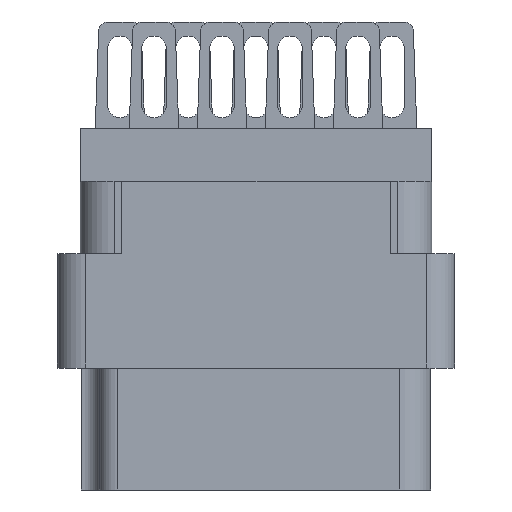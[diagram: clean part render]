
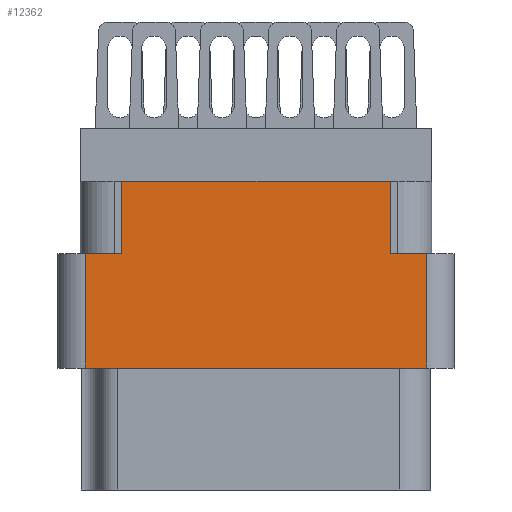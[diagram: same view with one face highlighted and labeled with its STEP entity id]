
A CAD part, left-side view. The second image highlights one B-rep face of the part: STEP entity #12362.
In plain terms, the highlighted planar face has unit normal (-1, 0, 0).
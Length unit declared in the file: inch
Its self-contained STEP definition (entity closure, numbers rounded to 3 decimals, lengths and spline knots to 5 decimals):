
#1433 = CARTESIAN_POINT ( 'NONE',  ( -1.296, 0., -0.277 ) ) ;
#1527 = VECTOR ( 'NONE', #34134, 39.37008 ) ;
#1602 = ORIENTED_EDGE ( 'NONE', *, *, #22828, .F. ) ;
#4025 = VECTOR ( 'NONE', #23517, 39.37008 ) ;
#4222 = DIRECTION ( 'NONE',  ( 0., -1., 0. ) ) ;
#6904 = VERTEX_POINT ( 'NONE', #41774 ) ;
#7557 = ORIENTED_EDGE ( 'NONE', *, *, #26108, .F. ) ;
#8446 = DIRECTION ( 'NONE',  ( -1., 0., 0. ) ) ;
#8701 = DIRECTION ( 'NONE',  ( 0., -1., 0. ) ) ;
#10532 = CARTESIAN_POINT ( 'NONE',  ( -1.296, 0.296, -0.277 ) ) ;
#11224 = LINE ( 'NONE', #1433, #1527 ) ;
#11901 = CARTESIAN_POINT ( 'NONE',  ( -1.296, -0.296, -0.117 ) ) ;
#12362 = ADVANCED_FACE ( 'NONE', ( #31519 ), #41620, .T. ) ;
#13215 = VECTOR ( 'NONE', #15807, 39.37008 ) ;
#15366 = EDGE_CURVE ( 'NONE', #37491, #18686, #37211, .T. ) ;
#15807 = DIRECTION ( 'NONE',  ( 0., 0., 1. ) ) ;
#16629 = ORIENTED_EDGE ( 'NONE', *, *, #15366, .T. ) ;
#18030 = ORIENTED_EDGE ( 'NONE', *, *, #46895, .F. ) ;
#18686 = VERTEX_POINT ( 'NONE', #47164 ) ;
#18992 = CARTESIAN_POINT ( 'NONE',  ( -1.296, 0.438, -0.117 ) ) ;
#20115 = VERTEX_POINT ( 'NONE', #20280 ) ;
#20280 = CARTESIAN_POINT ( 'NONE',  ( -1.296, -0.376, -0.529 ) ) ;
#20473 = LINE ( 'NONE', #41917, #4025 ) ;
#21093 = LINE ( 'NONE', #18992, #23906 ) ;
#21752 = CARTESIAN_POINT ( 'NONE',  ( -1.296, 0.296, -0.117 ) ) ;
#22828 = EDGE_CURVE ( 'NONE', #41515, #23823, #27057, .T. ) ;
#23211 = CARTESIAN_POINT ( 'NONE',  ( -1.296, -0.376, -0.277 ) ) ;
#23517 = DIRECTION ( 'NONE',  ( 0., 0., 1. ) ) ;
#23823 = VERTEX_POINT ( 'NONE', #21752 ) ;
#23906 = VECTOR ( 'NONE', #4222, 39.37008 ) ;
#25377 = ORIENTED_EDGE ( 'NONE', *, *, #26631, .T. ) ;
#26108 = EDGE_CURVE ( 'NONE', #37491, #41515, #35412, .T. ) ;
#26454 = VERTEX_POINT ( 'NONE', #23211 ) ;
#26631 = EDGE_CURVE ( 'NONE', #6904, #33984, #20473, .T. ) ;
#27057 = LINE ( 'NONE', #27490, #40815 ) ;
#27490 = CARTESIAN_POINT ( 'NONE',  ( -1.296, 0.296, -0.277 ) ) ;
#27792 = DIRECTION ( 'NONE',  ( 0., 0., -1. ) ) ;
#29045 = ORIENTED_EDGE ( 'NONE', *, *, #40742, .T. ) ;
#29537 = EDGE_CURVE ( 'NONE', #23823, #33984, #21093, .T. ) ;
#29660 = CARTESIAN_POINT ( 'NONE',  ( -1.296, -0.376, -0.798 ) ) ;
#30866 = VECTOR ( 'NONE', #27792, 39.37008 ) ;
#31105 = DIRECTION ( 'NONE',  ( 0., 1., 0. ) ) ;
#31111 = CARTESIAN_POINT ( 'NONE',  ( -1.296, 0., -0.277 ) ) ;
#31151 = DIRECTION ( 'NONE',  ( 0., 0., 1. ) ) ;
#31294 = AXIS2_PLACEMENT_3D ( 'NONE', #41465, #8446, #33954 ) ;
#31519 = FACE_OUTER_BOUND ( 'NONE', #43573, .T. ) ;
#32199 = LINE ( 'NONE', #38674, #34525 ) ;
#32902 = EDGE_CURVE ( 'NONE', #20115, #18686, #32199, .T. ) ;
#33954 = DIRECTION ( 'NONE',  ( 0., 0., 1. ) ) ;
#33984 = VERTEX_POINT ( 'NONE', #11901 ) ;
#34134 = DIRECTION ( 'NONE',  ( 0., -1., 0. ) ) ;
#34525 = VECTOR ( 'NONE', #31105, 39.37008 ) ;
#35412 = LINE ( 'NONE', #31111, #37161 ) ;
#37161 = VECTOR ( 'NONE', #8701, 39.37008 ) ;
#37211 = LINE ( 'NONE', #39186, #30866 ) ;
#37491 = VERTEX_POINT ( 'NONE', #44864 ) ;
#38674 = CARTESIAN_POINT ( 'NONE',  ( -1.296, 0., -0.529 ) ) ;
#39186 = CARTESIAN_POINT ( 'NONE',  ( -1.296, 0.376, -0.798 ) ) ;
#40742 = EDGE_CURVE ( 'NONE', #20115, #26454, #42381, .T. ) ;
#40815 = VECTOR ( 'NONE', #31151, 39.37008 ) ;
#41465 = CARTESIAN_POINT ( 'NONE',  ( -1.296, -0.438, -0.798 ) ) ;
#41515 = VERTEX_POINT ( 'NONE', #10532 ) ;
#41620 = PLANE ( 'NONE',  #31294 ) ;
#41774 = CARTESIAN_POINT ( 'NONE',  ( -1.296, -0.296, -0.277 ) ) ;
#41917 = CARTESIAN_POINT ( 'NONE',  ( -1.296, -0.296, -0.277 ) ) ;
#42381 = LINE ( 'NONE', #29660, #13215 ) ;
#43460 = ORIENTED_EDGE ( 'NONE', *, *, #32902, .F. ) ;
#43573 = EDGE_LOOP ( 'NONE', ( #7557, #16629, #43460, #29045, #18030, #25377, #45716, #1602 ) ) ;
#44864 = CARTESIAN_POINT ( 'NONE',  ( -1.296, 0.376, -0.277 ) ) ;
#45716 = ORIENTED_EDGE ( 'NONE', *, *, #29537, .F. ) ;
#46895 = EDGE_CURVE ( 'NONE', #6904, #26454, #11224, .T. ) ;
#47164 = CARTESIAN_POINT ( 'NONE',  ( -1.296, 0.376, -0.529 ) ) ;
